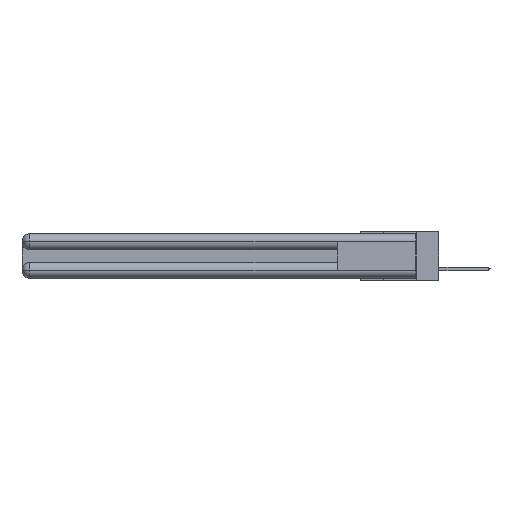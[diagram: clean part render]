
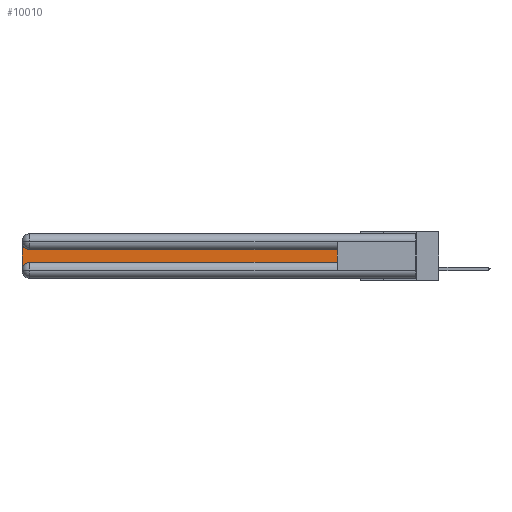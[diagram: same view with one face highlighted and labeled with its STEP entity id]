
A CAD part, left-side view. The second image highlights one B-rep face of the part: STEP entity #10010.
In plain terms, the highlighted planar face has unit normal (-1, 0, 0).
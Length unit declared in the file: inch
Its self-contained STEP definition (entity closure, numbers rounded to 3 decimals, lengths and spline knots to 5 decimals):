
#685 = VERTEX_POINT ( 'NONE', #26533 ) ;
#1597 = VERTEX_POINT ( 'NONE', #11124 ) ;
#5245 = DIRECTION ( 'NONE',  ( 0., 1., 0. ) ) ;
#5252 = AXIS2_PLACEMENT_3D ( 'NONE', #22709, #11244, #27941 ) ;
#5808 = ORIENTED_EDGE ( 'NONE', *, *, #17331, .T. ) ;
#6102 = CIRCLE ( 'NONE', #5252, 0.06 ) ;
#6310 = DIRECTION ( 'NONE',  ( 0., 0., -1. ) ) ;
#7449 = CARTESIAN_POINT ( 'NONE',  ( 0.075, 0.6, -0.2175 ) ) ;
#7743 = CARTESIAN_POINT ( 'NONE',  ( 0.075, 0.6, -0.1225 ) ) ;
#7808 = LINE ( 'NONE', #7743, #26114 ) ;
#8503 = ORIENTED_EDGE ( 'NONE', *, *, #13258, .T. ) ;
#8611 = EDGE_LOOP ( 'NONE', ( #23342, #27612, #22814, #8503, #5808, #28522 ) ) ;
#8855 = VERTEX_POINT ( 'NONE', #19092 ) ;
#9405 = EDGE_CURVE ( 'NONE', #14738, #1597, #10748, .T. ) ;
#9737 = VECTOR ( 'NONE', #29649, 39.37008 ) ;
#9985 = AXIS2_PLACEMENT_3D ( 'NONE', #13443, #13750, #16036 ) ;
#10010 = ADVANCED_FACE ( 'NONE', ( #27913 ), #27847, .F. ) ;
#10748 = LINE ( 'NONE', #13413, #12279 ) ;
#10818 = CARTESIAN_POINT ( 'NONE',  ( 0.075, 2.94, -0.0625 ) ) ;
#11124 = CARTESIAN_POINT ( 'NONE',  ( 0.075, 3., -0.2775 ) ) ;
#11244 = DIRECTION ( 'NONE',  ( 1., 0., 0. ) ) ;
#11286 = CARTESIAN_POINT ( 'NONE',  ( 0.075, 2.94, -0.1225 ) ) ;
#12226 = VECTOR ( 'NONE', #26354, 39.37008 ) ;
#12279 = VECTOR ( 'NONE', #6310, 39.37008 ) ;
#12604 = DIRECTION ( 'NONE',  ( 1., 0., 0. ) ) ;
#12954 = CARTESIAN_POINT ( 'NONE',  ( 0.075, 0.6, -0.2175 ) ) ;
#13127 = DIRECTION ( 'NONE',  ( 0., 0., -1. ) ) ;
#13258 = EDGE_CURVE ( 'NONE', #1597, #685, #6102, .T. ) ;
#13413 = CARTESIAN_POINT ( 'NONE',  ( 0.075, 3., -0.2175 ) ) ;
#13443 = CARTESIAN_POINT ( 'NONE',  ( 0.075, 3., -0.1225 ) ) ;
#13750 = DIRECTION ( 'NONE',  ( 1., 0., 0. ) ) ;
#14738 = VERTEX_POINT ( 'NONE', #19160 ) ;
#15061 = VERTEX_POINT ( 'NONE', #11286 ) ;
#15479 = EDGE_CURVE ( 'NONE', #26470, #8855, #23569, .T. ) ;
#16036 = DIRECTION ( 'NONE',  ( 0., 0., -1. ) ) ;
#16962 = AXIS2_PLACEMENT_3D ( 'NONE', #10818, #12604, #13127 ) ;
#17331 = EDGE_CURVE ( 'NONE', #685, #26470, #18562, .T. ) ;
#17845 = CARTESIAN_POINT ( 'NONE',  ( 0.075, 0.6, -0.2175 ) ) ;
#18562 = LINE ( 'NONE', #7449, #12226 ) ;
#19092 = CARTESIAN_POINT ( 'NONE',  ( 0.075, 0.6, -0.1225 ) ) ;
#19160 = CARTESIAN_POINT ( 'NONE',  ( 0.075, 3., -0.0625 ) ) ;
#22129 = CIRCLE ( 'NONE', #16962, 0.06 ) ;
#22709 = CARTESIAN_POINT ( 'NONE',  ( 0.075, 2.94, -0.2775 ) ) ;
#22814 = ORIENTED_EDGE ( 'NONE', *, *, #9405, .T. ) ;
#23342 = ORIENTED_EDGE ( 'NONE', *, *, #26341, .T. ) ;
#23569 = LINE ( 'NONE', #17845, #9737 ) ;
#26114 = VECTOR ( 'NONE', #5245, 39.37008 ) ;
#26341 = EDGE_CURVE ( 'NONE', #8855, #15061, #7808, .T. ) ;
#26354 = DIRECTION ( 'NONE',  ( 0., -1., 0. ) ) ;
#26470 = VERTEX_POINT ( 'NONE', #12954 ) ;
#26533 = CARTESIAN_POINT ( 'NONE',  ( 0.075, 2.94, -0.2175 ) ) ;
#27612 = ORIENTED_EDGE ( 'NONE', *, *, #30786, .T. ) ;
#27847 = PLANE ( 'NONE',  #9985 ) ;
#27913 = FACE_OUTER_BOUND ( 'NONE', #8611, .T. ) ;
#27941 = DIRECTION ( 'NONE',  ( 0., 0., -1. ) ) ;
#28522 = ORIENTED_EDGE ( 'NONE', *, *, #15479, .T. ) ;
#29649 = DIRECTION ( 'NONE',  ( 0., 0., 1. ) ) ;
#30786 = EDGE_CURVE ( 'NONE', #15061, #14738, #22129, .T. ) ;
